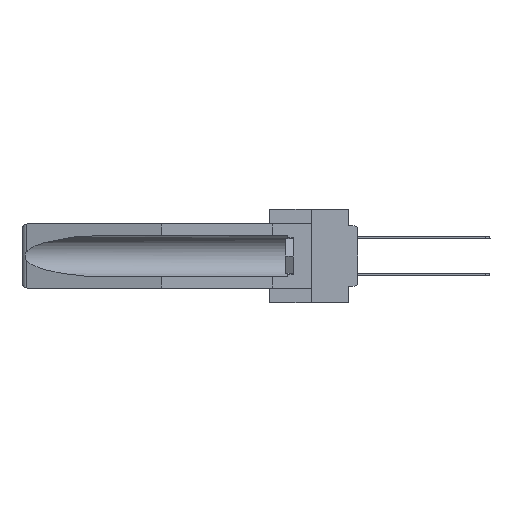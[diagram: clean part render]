
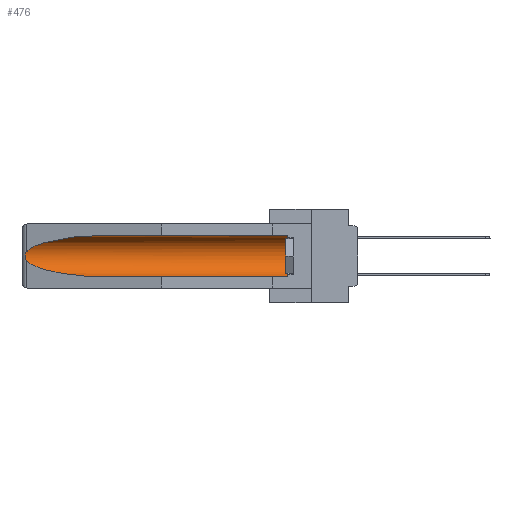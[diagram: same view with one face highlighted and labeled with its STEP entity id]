
A CAD part, left-side view. The second image highlights one B-rep face of the part: STEP entity #476.
In plain terms, the highlighted cylindrical face has radius 2.857 mm (diameter 5.715 mm), a partial arc.
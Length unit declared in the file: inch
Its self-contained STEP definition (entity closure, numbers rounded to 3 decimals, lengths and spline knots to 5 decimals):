
#9 = CARTESIAN_POINT ( 'NONE',  ( 0.25451, 1.48313, -0.24835 ) ) ;
#167 = AXIS2_PLACEMENT_3D ( 'NONE', #6232, #11915, #17358 ) ;
#319 = CARTESIAN_POINT ( 'NONE',  ( 0.21114, 1.30732, -0.059 ) ) ;
#476 = ADVANCED_FACE ( 'NONE', ( #34442 ), #11908, .F. ) ;
#1278 = CARTESIAN_POINT ( 'NONE',  ( 0.26655, 1.53094, -0.18657 ) ) ;
#2919 = CARTESIAN_POINT ( 'NONE',  ( 0.155, 0.126, -0.059 ) ) ;
#4197 = CARTESIAN_POINT ( 'NONE',  ( 0.2673, 1.53269, -0.17917 ) ) ;
#5973 = EDGE_CURVE ( 'NONE', #17975, #29799, #20056, .T. ) ;
#6232 = CARTESIAN_POINT ( 'NONE',  ( 0.155, 0.126, -0.1715 ) ) ;
#7336 = CARTESIAN_POINT ( 'NONE',  ( 0.26537, 1.52718, -0.19328 ) ) ;
#7464 = CARTESIAN_POINT ( 'NONE',  ( 0.2675, 1.53308, -0.17534 ) ) ;
#7768 = ORIENTED_EDGE ( 'NONE', *, *, #23652, .T. ) ;
#8334 = CARTESIAN_POINT ( 'NONE',  ( 0.26537, 1.52718, -0.14972 ) ) ;
#9479 = CIRCLE ( 'NONE', #167, 0.1125 ) ;
#9893 = DIRECTION ( 'NONE',  ( 0., 1., 0. ) ) ;
#10192 = VECTOR ( 'NONE', #28419, 39.37008 ) ;
#10283 = B_SPLINE_CURVE_WITH_KNOTS ( 'NONE', 3,
 ( #32061, #26436, #20965, #32429, #18219, #7464, #4197, #1278, #18040, #26783 ),
 .UNSPECIFIED., .F., .F.,
 ( 4, 2, 2, 2, 4 ),
 ( 0., 0.00029, 0.00058, 0.00087, 0.00117 ),
 .UNSPECIFIED. ) ;
#10582 = CARTESIAN_POINT ( 'NONE',  ( 0.155, 1.07973, -0.059 ) ) ;
#10700 =( BOUNDED_CURVE ( )  B_SPLINE_CURVE ( 3, ( #7336, #9, #11141, #21015 ),
 .UNSPECIFIED., .F., .F. ) 
 B_SPLINE_CURVE_WITH_KNOTS ( ( 4, 4 ),
 ( 0.1948, 1.5708 ),
 .UNSPECIFIED. ) 
 CURVE ( )  GEOMETRIC_REPRESENTATION_ITEM ( )  RATIONAL_B_SPLINE_CURVE ( ( 1., 0.848, 0.848, 1. ) ) 
 REPRESENTATION_ITEM ( '' )  );
#11141 = CARTESIAN_POINT ( 'NONE',  ( 0.21114, 1.30732, -0.284 ) ) ;
#11678 = EDGE_CURVE ( 'NONE', #29239, #32597, #10700, .T. ) ;
#11908 = CYLINDRICAL_SURFACE ( 'NONE', #21485, 0.1125 ) ;
#11915 = DIRECTION ( 'NONE',  ( 0., -1., 0. ) ) ;
#13572 = CARTESIAN_POINT ( 'NONE',  ( 0.155, 0.126, -0.284 ) ) ;
#14805 = ORIENTED_EDGE ( 'NONE', *, *, #21828, .F. ) ;
#14822 = CARTESIAN_POINT ( 'NONE',  ( 0.26537, 1.52718, -0.19328 ) ) ;
#15531 = CARTESIAN_POINT ( 'NONE',  ( 0.155, 1.07973, -0.284 ) ) ;
#17182 = ORIENTED_EDGE ( 'NONE', *, *, #17419, .T. ) ;
#17320 = CARTESIAN_POINT ( 'NONE',  ( 0.155, -0.30754, -0.059 ) ) ;
#17350 = CARTESIAN_POINT ( 'NONE',  ( 0.155, -0.30754, -0.1715 ) ) ;
#17358 = DIRECTION ( 'NONE',  ( 0., 0., 1. ) ) ;
#17419 = EDGE_CURVE ( 'NONE', #32271, #17975, #9479, .T. ) ;
#17975 = VERTEX_POINT ( 'NONE', #2919 ) ;
#18040 = CARTESIAN_POINT ( 'NONE',  ( 0.26597, 1.5296, -0.19026 ) ) ;
#18219 = CARTESIAN_POINT ( 'NONE',  ( 0.2675, 1.53308, -0.16763 ) ) ;
#18440 = EDGE_CURVE ( 'NONE', #29799, #27028, #20457, .T. ) ;
#20056 = LINE ( 'NONE', #17320, #10192 ) ;
#20457 =( BOUNDED_CURVE ( )  B_SPLINE_CURVE ( 3, ( #30555, #319, #25099, #8334 ),
 .UNSPECIFIED., .F., .F. ) 
 B_SPLINE_CURVE_WITH_KNOTS ( ( 4, 4 ),
 ( 4.71239, 6.08839 ),
 .UNSPECIFIED. ) 
 CURVE ( )  GEOMETRIC_REPRESENTATION_ITEM ( )  RATIONAL_B_SPLINE_CURVE ( ( 1., 0.848, 0.848, 1. ) ) 
 REPRESENTATION_ITEM ( '' )  );
#20965 = CARTESIAN_POINT ( 'NONE',  ( 0.26654, 1.53092, -0.15636 ) ) ;
#21015 = CARTESIAN_POINT ( 'NONE',  ( 0.155, 1.07973, -0.284 ) ) ;
#21021 = EDGE_LOOP ( 'NONE', ( #24763, #7768, #22958, #14805, #17182, #30056 ) ) ;
#21485 = AXIS2_PLACEMENT_3D ( 'NONE', #17350, #28275, #28632 ) ;
#21828 = EDGE_CURVE ( 'NONE', #32271, #32597, #24270, .T. ) ;
#22958 = ORIENTED_EDGE ( 'NONE', *, *, #11678, .T. ) ;
#23652 = EDGE_CURVE ( 'NONE', #27028, #29239, #10283, .T. ) ;
#24270 = LINE ( 'NONE', #26635, #31532 ) ;
#24763 = ORIENTED_EDGE ( 'NONE', *, *, #18440, .T. ) ;
#25099 = CARTESIAN_POINT ( 'NONE',  ( 0.25451, 1.48313, -0.09465 ) ) ;
#26436 = CARTESIAN_POINT ( 'NONE',  ( 0.26597, 1.52961, -0.15275 ) ) ;
#26635 = CARTESIAN_POINT ( 'NONE',  ( 0.155, -0.30754, -0.284 ) ) ;
#26783 = CARTESIAN_POINT ( 'NONE',  ( 0.26537, 1.52718, -0.19328 ) ) ;
#27028 = VERTEX_POINT ( 'NONE', #27833 ) ;
#27833 = CARTESIAN_POINT ( 'NONE',  ( 0.26537, 1.52718, -0.14972 ) ) ;
#28275 = DIRECTION ( 'NONE',  ( 0., 1., 0. ) ) ;
#28419 = DIRECTION ( 'NONE',  ( 0., 1., 0. ) ) ;
#28632 = DIRECTION ( 'NONE',  ( 0., 0., 1. ) ) ;
#29239 = VERTEX_POINT ( 'NONE', #14822 ) ;
#29799 = VERTEX_POINT ( 'NONE', #10582 ) ;
#30056 = ORIENTED_EDGE ( 'NONE', *, *, #5973, .T. ) ;
#30555 = CARTESIAN_POINT ( 'NONE',  ( 0.155, 1.07973, -0.059 ) ) ;
#31532 = VECTOR ( 'NONE', #9893, 39.37008 ) ;
#32061 = CARTESIAN_POINT ( 'NONE',  ( 0.26537, 1.52718, -0.14972 ) ) ;
#32271 = VERTEX_POINT ( 'NONE', #13572 ) ;
#32429 = CARTESIAN_POINT ( 'NONE',  ( 0.2673, 1.5327, -0.16383 ) ) ;
#32597 = VERTEX_POINT ( 'NONE', #15531 ) ;
#34442 = FACE_OUTER_BOUND ( 'NONE', #21021, .T. ) ;
